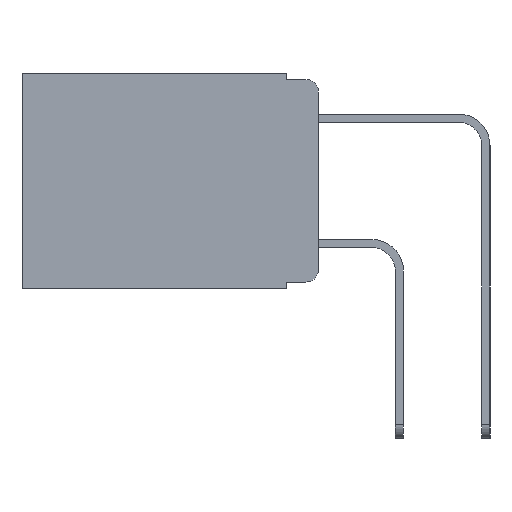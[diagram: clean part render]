
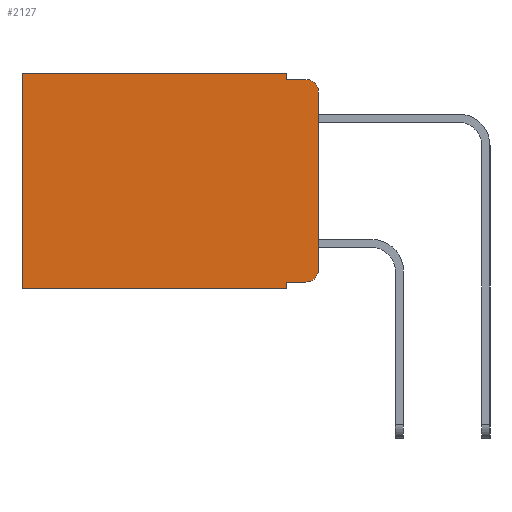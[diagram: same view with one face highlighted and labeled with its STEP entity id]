
A CAD part, left-side view. The second image highlights one B-rep face of the part: STEP entity #2127.
In plain terms, the highlighted planar face has unit normal (-1, 0, 0).
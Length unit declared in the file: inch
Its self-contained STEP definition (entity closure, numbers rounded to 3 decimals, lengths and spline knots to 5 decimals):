
#47 = EDGE_CURVE ( 'NONE', #14373, #13072, #1173, .T. ) ;
#528 = CARTESIAN_POINT ( 'NONE',  ( 0.298, 0., -0.313 ) ) ;
#562 = VECTOR ( 'NONE', #4478, 39.37008 ) ;
#839 = EDGE_CURVE ( 'NONE', #10723, #4140, #2711, .T. ) ;
#1072 = EDGE_CURVE ( 'NONE', #3563, #10723, #5743, .T. ) ;
#1114 = VECTOR ( 'NONE', #13814, 39.37008 ) ;
#1173 = LINE ( 'NONE', #10801, #13390 ) ;
#1656 = EDGE_CURVE ( 'NONE', #3563, #7736, #3847, .T. ) ;
#1936 = LINE ( 'NONE', #10401, #13728 ) ;
#2127 = ADVANCED_FACE ( 'NONE', ( #12800 ), #3024, .F. ) ;
#2281 = CARTESIAN_POINT ( 'NONE',  ( 0.298, 0.051, -0.01 ) ) ;
#2633 = ORIENTED_EDGE ( 'NONE', *, *, #12278, .T. ) ;
#2711 = LINE ( 'NONE', #13967, #9091 ) ;
#2714 = ORIENTED_EDGE ( 'NONE', *, *, #47, .F. ) ;
#2745 = ORIENTED_EDGE ( 'NONE', *, *, #839, .T. ) ;
#2804 = ORIENTED_EDGE ( 'NONE', *, *, #1656, .F. ) ;
#2893 = ORIENTED_EDGE ( 'NONE', *, *, #4965, .T. ) ;
#2951 = ORIENTED_EDGE ( 'NONE', *, *, #8166, .F. ) ;
#3024 = PLANE ( 'NONE',  #3816 ) ;
#3282 = DIRECTION ( 'NONE',  ( -1., 0., 0. ) ) ;
#3301 = DIRECTION ( 'NONE',  ( 0., 0., -1. ) ) ;
#3314 = DIRECTION ( 'NONE',  ( 1., 0., 0. ) ) ;
#3324 = EDGE_CURVE ( 'NONE', #7736, #11457, #8833, .T. ) ;
#3350 = DIRECTION ( 'NONE',  ( 0., 0., -1. ) ) ;
#3563 = VERTEX_POINT ( 'NONE', #8051 ) ;
#3816 = AXIS2_PLACEMENT_3D ( 'NONE', #5726, #3314, #3301 ) ;
#3826 = VERTEX_POINT ( 'NONE', #11779 ) ;
#3847 = LINE ( 'NONE', #4489, #562 ) ;
#4128 = DIRECTION ( 'NONE',  ( 0., 1., 0. ) ) ;
#4140 = VERTEX_POINT ( 'NONE', #11018 ) ;
#4459 = LINE ( 'NONE', #5245, #13385 ) ;
#4472 = ORIENTED_EDGE ( 'NONE', *, *, #13809, .T. ) ;
#4478 = DIRECTION ( 'NONE',  ( 0., 0., -1. ) ) ;
#4489 = CARTESIAN_POINT ( 'NONE',  ( 0.298, 0.051, 0. ) ) ;
#4965 = EDGE_CURVE ( 'NONE', #9494, #11457, #7745, .T. ) ;
#5025 = ORIENTED_EDGE ( 'NONE', *, *, #12688, .F. ) ;
#5245 = CARTESIAN_POINT ( 'NONE',  ( 0.298, 0., -0.343 ) ) ;
#5672 = VECTOR ( 'NONE', #8400, 39.37008 ) ;
#5722 = CARTESIAN_POINT ( 'NONE',  ( 0.298, 0.051, -0.333 ) ) ;
#5726 = CARTESIAN_POINT ( 'NONE',  ( 0.298, 0., 0. ) ) ;
#5743 = LINE ( 'NONE', #7472, #8541 ) ;
#5993 = ORIENTED_EDGE ( 'NONE', *, *, #1072, .T. ) ;
#6029 = AXIS2_PLACEMENT_3D ( 'NONE', #7466, #10231, #10146 ) ;
#6730 = ORIENTED_EDGE ( 'NONE', *, *, #3324, .F. ) ;
#7218 = LINE ( 'NONE', #5722, #1114 ) ;
#7466 = CARTESIAN_POINT ( 'NONE',  ( 0.298, 0.02, -0.03 ) ) ;
#7472 = CARTESIAN_POINT ( 'NONE',  ( 0.298, 0., 0. ) ) ;
#7736 = VERTEX_POINT ( 'NONE', #2281 ) ;
#7745 = CIRCLE ( 'NONE', #6029, 0.02 ) ;
#8051 = CARTESIAN_POINT ( 'NONE',  ( 0.298, 0.051, 0. ) ) ;
#8166 = EDGE_CURVE ( 'NONE', #9494, #14281, #1936, .T. ) ;
#8400 = DIRECTION ( 'NONE',  ( 0., -1., 0. ) ) ;
#8541 = VECTOR ( 'NONE', #4128, 39.37008 ) ;
#8833 = LINE ( 'NONE', #12132, #5672 ) ;
#9091 = VECTOR ( 'NONE', #11611, 39.37008 ) ;
#9457 = DIRECTION ( 'NONE',  ( 0., 0., -1. ) ) ;
#9494 = VERTEX_POINT ( 'NONE', #10713 ) ;
#9790 = CIRCLE ( 'NONE', #13778, 0.02 ) ;
#10146 = DIRECTION ( 'NONE',  ( 0., 0., -1. ) ) ;
#10231 = DIRECTION ( 'NONE',  ( -1., 0., 0. ) ) ;
#10270 = CARTESIAN_POINT ( 'NONE',  ( 0.298, 0.051, -0.333 ) ) ;
#10349 = CARTESIAN_POINT ( 'NONE',  ( 0.298, 0.02, -0.313 ) ) ;
#10401 = CARTESIAN_POINT ( 'NONE',  ( 0.298, 0., 0. ) ) ;
#10713 = CARTESIAN_POINT ( 'NONE',  ( 0.298, 0., -0.03 ) ) ;
#10723 = VERTEX_POINT ( 'NONE', #11869 ) ;
#10801 = CARTESIAN_POINT ( 'NONE',  ( 0.298, 0.051, 0. ) ) ;
#11018 = CARTESIAN_POINT ( 'NONE',  ( 0.298, 0.473, -0.343 ) ) ;
#11044 = DIRECTION ( 'NONE',  ( 0., 1., 0. ) ) ;
#11457 = VERTEX_POINT ( 'NONE', #14380 ) ;
#11510 = DIRECTION ( 'NONE',  ( 0., 0., -1. ) ) ;
#11611 = DIRECTION ( 'NONE',  ( 0., 0., -1. ) ) ;
#11779 = CARTESIAN_POINT ( 'NONE',  ( 0.298, 0.02, -0.333 ) ) ;
#11810 = CARTESIAN_POINT ( 'NONE',  ( 0.298, 0.051, -0.343 ) ) ;
#11869 = CARTESIAN_POINT ( 'NONE',  ( 0.298, 0.473, 0. ) ) ;
#12132 = CARTESIAN_POINT ( 'NONE',  ( 0.298, 0.051, -0.01 ) ) ;
#12278 = EDGE_CURVE ( 'NONE', #3826, #14281, #9790, .T. ) ;
#12468 = EDGE_LOOP ( 'NONE', ( #2951, #2893, #6730, #2804, #5993, #2745, #5025, #2714, #4472, #2633 ) ) ;
#12688 = EDGE_CURVE ( 'NONE', #13072, #4140, #4459, .T. ) ;
#12800 = FACE_OUTER_BOUND ( 'NONE', #12468, .T. ) ;
#13072 = VERTEX_POINT ( 'NONE', #11810 ) ;
#13385 = VECTOR ( 'NONE', #11044, 39.37008 ) ;
#13390 = VECTOR ( 'NONE', #9457, 39.37008 ) ;
#13728 = VECTOR ( 'NONE', #3350, 39.37008 ) ;
#13778 = AXIS2_PLACEMENT_3D ( 'NONE', #10349, #3282, #11510 ) ;
#13809 = EDGE_CURVE ( 'NONE', #14373, #3826, #7218, .T. ) ;
#13814 = DIRECTION ( 'NONE',  ( 0., -1., 0. ) ) ;
#13967 = CARTESIAN_POINT ( 'NONE',  ( 0.298, 0.473, 0. ) ) ;
#14281 = VERTEX_POINT ( 'NONE', #528 ) ;
#14373 = VERTEX_POINT ( 'NONE', #10270 ) ;
#14380 = CARTESIAN_POINT ( 'NONE',  ( 0.298, 0.02, -0.01 ) ) ;
